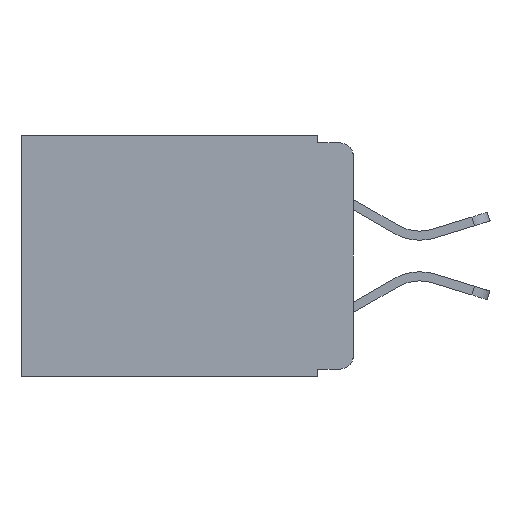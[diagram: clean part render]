
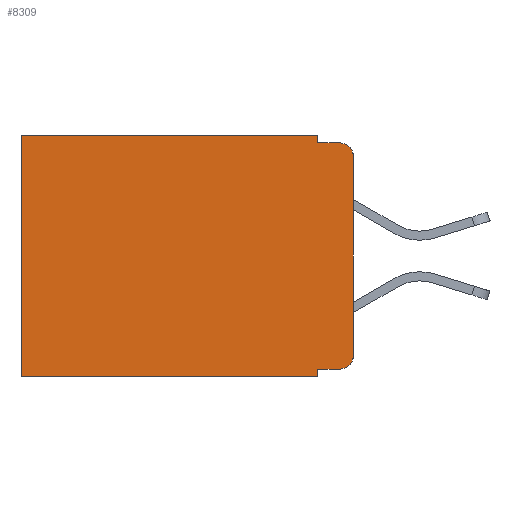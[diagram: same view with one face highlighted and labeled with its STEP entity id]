
A CAD part, left-side view. The second image highlights one B-rep face of the part: STEP entity #8309.
In plain terms, the highlighted planar face has unit normal (-1, 0, 0).
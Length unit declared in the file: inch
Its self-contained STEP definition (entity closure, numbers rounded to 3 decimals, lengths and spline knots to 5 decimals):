
#271 = CARTESIAN_POINT ( 'NONE',  ( 0.298, 0.051, -0.343 ) ) ;
#281 = DIRECTION ( 'NONE',  ( 0., 1., 0. ) ) ;
#534 = CIRCLE ( 'NONE', #15281, 0.02 ) ;
#556 = AXIS2_PLACEMENT_3D ( 'NONE', #9745, #11533, #9820 ) ;
#1014 = CARTESIAN_POINT ( 'NONE',  ( 0.298, 0.051, 0. ) ) ;
#1052 = EDGE_CURVE ( 'NONE', #3668, #14519, #10321, .T. ) ;
#1294 = DIRECTION ( 'NONE',  ( 0., 0., -1. ) ) ;
#1438 = CARTESIAN_POINT ( 'NONE',  ( 0.298, 0.473, 0. ) ) ;
#1562 = LINE ( 'NONE', #1438, #22107 ) ;
#1724 = CARTESIAN_POINT ( 'NONE',  ( 0.298, 0.051, -0.01 ) ) ;
#1822 = CARTESIAN_POINT ( 'NONE',  ( 0.298, 0., -0.343 ) ) ;
#1970 = EDGE_CURVE ( 'NONE', #3668, #9273, #7495, .T. ) ;
#2002 = EDGE_LOOP ( 'NONE', ( #8130, #22467, #21306, #2809, #8905, #7438, #13604, #20705, #5360, #19246 ) ) ;
#2632 = LINE ( 'NONE', #1724, #11154 ) ;
#2663 = CARTESIAN_POINT ( 'NONE',  ( 0.298, 0., -0.313 ) ) ;
#2809 = ORIENTED_EDGE ( 'NONE', *, *, #3739, .F. ) ;
#2869 = CARTESIAN_POINT ( 'NONE',  ( 0.298, 0., 0. ) ) ;
#3258 = DIRECTION ( 'NONE',  ( 0., -1., 0. ) ) ;
#3668 = VERTEX_POINT ( 'NONE', #4749 ) ;
#3693 = DIRECTION ( 'NONE',  ( 0., 0., -1. ) ) ;
#3739 = EDGE_CURVE ( 'NONE', #7104, #9336, #14032, .T. ) ;
#4382 = VERTEX_POINT ( 'NONE', #10843 ) ;
#4384 = VECTOR ( 'NONE', #281, 39.37008 ) ;
#4667 = EDGE_CURVE ( 'NONE', #14519, #8042, #19932, .T. ) ;
#4749 = CARTESIAN_POINT ( 'NONE',  ( 0.298, 0.051, -0.333 ) ) ;
#4755 = PLANE ( 'NONE',  #556 ) ;
#5269 = DIRECTION ( 'NONE',  ( 0., 0., -1. ) ) ;
#5360 = ORIENTED_EDGE ( 'NONE', *, *, #1970, .T. ) ;
#6206 = EDGE_CURVE ( 'NONE', #15896, #8042, #1562, .T. ) ;
#6878 = EDGE_CURVE ( 'NONE', #7104, #15896, #13589, .T. ) ;
#7013 = FACE_OUTER_BOUND ( 'NONE', #2002, .T. ) ;
#7104 = VERTEX_POINT ( 'NONE', #1014 ) ;
#7137 = CARTESIAN_POINT ( 'NONE',  ( 0.298, 0.051, 0. ) ) ;
#7438 = ORIENTED_EDGE ( 'NONE', *, *, #6206, .T. ) ;
#7495 = LINE ( 'NONE', #17311, #11914 ) ;
#8042 = VERTEX_POINT ( 'NONE', #22379 ) ;
#8130 = ORIENTED_EDGE ( 'NONE', *, *, #22590, .F. ) ;
#8309 = ADVANCED_FACE ( 'NONE', ( #7013 ), #4755, .F. ) ;
#8391 = VECTOR ( 'NONE', #3693, 39.37008 ) ;
#8393 = VECTOR ( 'NONE', #16435, 39.37008 ) ;
#8423 = CARTESIAN_POINT ( 'NONE',  ( 0.298, 0., -0.03 ) ) ;
#8587 = CARTESIAN_POINT ( 'NONE',  ( 0.298, 0.02, -0.333 ) ) ;
#8734 = CARTESIAN_POINT ( 'NONE',  ( 0.298, 0.051, 0. ) ) ;
#8905 = ORIENTED_EDGE ( 'NONE', *, *, #6878, .T. ) ;
#9090 = VERTEX_POINT ( 'NONE', #8423 ) ;
#9273 = VERTEX_POINT ( 'NONE', #8587 ) ;
#9336 = VERTEX_POINT ( 'NONE', #19569 ) ;
#9745 = CARTESIAN_POINT ( 'NONE',  ( 0.298, 0., 0. ) ) ;
#9820 = DIRECTION ( 'NONE',  ( 0., 0., -1. ) ) ;
#10321 = LINE ( 'NONE', #7137, #8391 ) ;
#10843 = CARTESIAN_POINT ( 'NONE',  ( 0.298, 0.02, -0.01 ) ) ;
#11134 = CARTESIAN_POINT ( 'NONE',  ( 0.298, 0., 0. ) ) ;
#11154 = VECTOR ( 'NONE', #3258, 39.37008 ) ;
#11362 = DIRECTION ( 'NONE',  ( -1., 0., 0. ) ) ;
#11533 = DIRECTION ( 'NONE',  ( 1., 0., 0. ) ) ;
#11914 = VECTOR ( 'NONE', #15182, 39.37008 ) ;
#12763 = EDGE_CURVE ( 'NONE', #9090, #4382, #534, .T. ) ;
#13094 = DIRECTION ( 'NONE',  ( 0., 0., -1. ) ) ;
#13565 = DIRECTION ( 'NONE',  ( 0., 0., -1. ) ) ;
#13589 = LINE ( 'NONE', #11134, #8393 ) ;
#13604 = ORIENTED_EDGE ( 'NONE', *, *, #4667, .F. ) ;
#14032 = LINE ( 'NONE', #8734, #17564 ) ;
#14519 = VERTEX_POINT ( 'NONE', #271 ) ;
#15182 = DIRECTION ( 'NONE',  ( 0., -1., 0. ) ) ;
#15251 = DIRECTION ( 'NONE',  ( 0., 0., -1. ) ) ;
#15281 = AXIS2_PLACEMENT_3D ( 'NONE', #16986, #22497, #15251 ) ;
#15896 = VERTEX_POINT ( 'NONE', #19579 ) ;
#15982 = LINE ( 'NONE', #2869, #16239 ) ;
#16158 = CIRCLE ( 'NONE', #18538, 0.02 ) ;
#16239 = VECTOR ( 'NONE', #13565, 39.37008 ) ;
#16435 = DIRECTION ( 'NONE',  ( 0., 1., 0. ) ) ;
#16986 = CARTESIAN_POINT ( 'NONE',  ( 0.298, 0.02, -0.03 ) ) ;
#17311 = CARTESIAN_POINT ( 'NONE',  ( 0.298, 0.051, -0.333 ) ) ;
#17564 = VECTOR ( 'NONE', #5269, 39.37008 ) ;
#18366 = EDGE_CURVE ( 'NONE', #9273, #19138, #16158, .T. ) ;
#18538 = AXIS2_PLACEMENT_3D ( 'NONE', #20074, #11362, #13094 ) ;
#19138 = VERTEX_POINT ( 'NONE', #2663 ) ;
#19246 = ORIENTED_EDGE ( 'NONE', *, *, #18366, .T. ) ;
#19569 = CARTESIAN_POINT ( 'NONE',  ( 0.298, 0.051, -0.01 ) ) ;
#19579 = CARTESIAN_POINT ( 'NONE',  ( 0.298, 0.473, 0. ) ) ;
#19932 = LINE ( 'NONE', #1822, #4384 ) ;
#20074 = CARTESIAN_POINT ( 'NONE',  ( 0.298, 0.02, -0.313 ) ) ;
#20705 = ORIENTED_EDGE ( 'NONE', *, *, #1052, .F. ) ;
#21306 = ORIENTED_EDGE ( 'NONE', *, *, #21709, .F. ) ;
#21709 = EDGE_CURVE ( 'NONE', #9336, #4382, #2632, .T. ) ;
#22107 = VECTOR ( 'NONE', #1294, 39.37008 ) ;
#22379 = CARTESIAN_POINT ( 'NONE',  ( 0.298, 0.473, -0.343 ) ) ;
#22467 = ORIENTED_EDGE ( 'NONE', *, *, #12763, .T. ) ;
#22497 = DIRECTION ( 'NONE',  ( -1., 0., 0. ) ) ;
#22590 = EDGE_CURVE ( 'NONE', #9090, #19138, #15982, .T. ) ;
